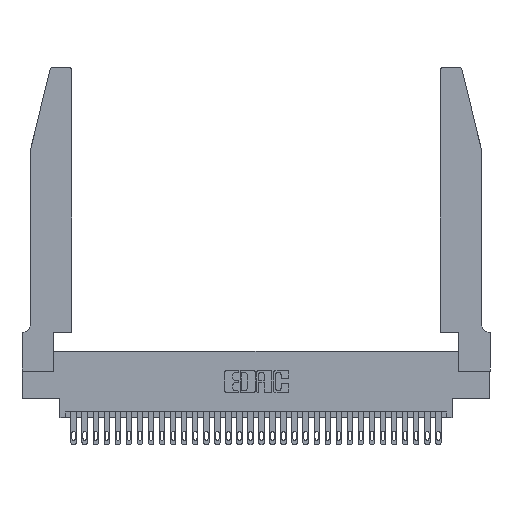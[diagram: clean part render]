
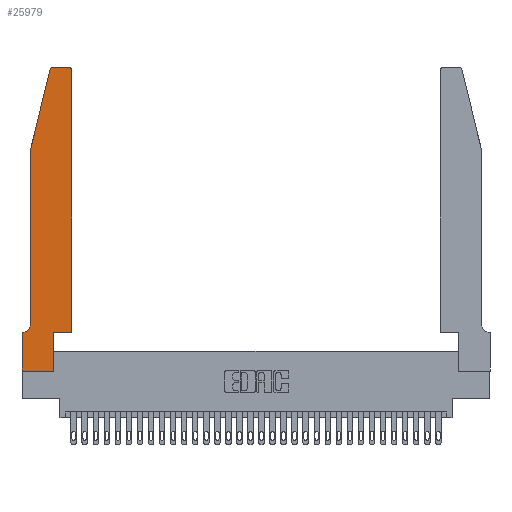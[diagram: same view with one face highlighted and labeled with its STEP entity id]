
A CAD part, top view. The second image highlights one B-rep face of the part: STEP entity #25979.
In plain terms, the highlighted planar face has unit normal (0, 0, 1).
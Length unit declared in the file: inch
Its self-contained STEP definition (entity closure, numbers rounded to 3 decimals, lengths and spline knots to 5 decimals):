
#18 = AXIS2_PLACEMENT_3D ( 'NONE', #23380, #5973, #31330 ) ;
#108 = CARTESIAN_POINT ( 'NONE',  ( 0., 0.35, 0.37 ) ) ;
#519 = VECTOR ( 'NONE', #17162, 39.37008 ) ;
#830 = EDGE_CURVE ( 'NONE', #32472, #28111, #31416, .T. ) ;
#1582 = CARTESIAN_POINT ( 'NONE',  ( 0.0755, 0.42, 0.37 ) ) ;
#1651 = CIRCLE ( 'NONE', #9747, 0.03 ) ;
#1728 = FACE_OUTER_BOUND ( 'NONE', #7332, .T. ) ;
#1952 = DIRECTION ( 'NONE',  ( -0.239, -0.971, 0. ) ) ;
#1981 = ORIENTED_EDGE ( 'NONE', *, *, #26642, .T. ) ;
#2197 = VECTOR ( 'NONE', #7999, 39.37008 ) ;
#3156 = DIRECTION ( 'NONE',  ( 1., 0., 0. ) ) ;
#3219 = VECTOR ( 'NONE', #1952, 39.37008 ) ;
#3643 = LINE ( 'NONE', #12323, #519 ) ;
#3748 = EDGE_CURVE ( 'NONE', #24625, #18290, #3643, .T. ) ;
#3863 = DIRECTION ( 'NONE',  ( 1., 0., 0. ) ) ;
#4399 = ORIENTED_EDGE ( 'NONE', *, *, #4541, .T. ) ;
#4404 = VECTOR ( 'NONE', #6775, 39.37008 ) ;
#4434 = CARTESIAN_POINT ( 'NONE',  ( 0.4205, 2.75, 0.37 ) ) ;
#4541 = EDGE_CURVE ( 'NONE', #13015, #24625, #31202, .T. ) ;
#5353 = DIRECTION ( 'NONE',  ( 1., 0., 0. ) ) ;
#5883 = AXIS2_PLACEMENT_3D ( 'NONE', #24911, #10011, #15133 ) ;
#5973 = DIRECTION ( 'NONE',  ( 0., 0., -1. ) ) ;
#6484 = LINE ( 'NONE', #19993, #23811 ) ;
#6775 = DIRECTION ( 'NONE',  ( -1., 0., 0. ) ) ;
#6852 = VERTEX_POINT ( 'NONE', #23525 ) ;
#6979 = LINE ( 'NONE', #23469, #15241 ) ;
#7052 = EDGE_CURVE ( 'NONE', #8730, #27240, #17762, .T. ) ;
#7332 = EDGE_LOOP ( 'NONE', ( #29798, #22419, #26788, #13953, #1981, #18088, #27158, #4399, #23398, #14567, #21724, #25975 ) ) ;
#7846 = CARTESIAN_POINT ( 'NONE',  ( 0., 0.35, 0.37 ) ) ;
#7999 = DIRECTION ( 'NONE',  ( 1., 0., 0. ) ) ;
#8064 = DIRECTION ( 'NONE',  ( 0., 0., 1. ) ) ;
#8126 = DIRECTION ( 'NONE',  ( 0., -1., 0. ) ) ;
#8561 = CARTESIAN_POINT ( 'NONE',  ( 0.0755, 0.35, 0.37 ) ) ;
#8730 = VERTEX_POINT ( 'NONE', #4434 ) ;
#9747 = AXIS2_PLACEMENT_3D ( 'NONE', #25950, #8064, #3156 ) ;
#10011 = DIRECTION ( 'NONE',  ( 0., 0., 1. ) ) ;
#11423 = EDGE_CURVE ( 'NONE', #18290, #19737, #23828, .T. ) ;
#12323 = CARTESIAN_POINT ( 'NONE',  ( 0.2865, 0.35, 0.37 ) ) ;
#12983 = CARTESIAN_POINT ( 'NONE',  ( 0.0755, 2., 0.37 ) ) ;
#13015 = VERTEX_POINT ( 'NONE', #13806 ) ;
#13100 = CARTESIAN_POINT ( 'NONE',  ( 0.0755, 2., 0.37 ) ) ;
#13135 = EDGE_CURVE ( 'NONE', #6852, #32472, #14250, .T. ) ;
#13806 = CARTESIAN_POINT ( 'NONE',  ( 0., 0., 0.37 ) ) ;
#13953 = ORIENTED_EDGE ( 'NONE', *, *, #830, .T. ) ;
#14250 = LINE ( 'NONE', #26693, #3219 ) ;
#14567 = ORIENTED_EDGE ( 'NONE', *, *, #11423, .T. ) ;
#14790 = CARTESIAN_POINT ( 'NONE',  ( 0.4505, 0.35, 0.37 ) ) ;
#15133 = DIRECTION ( 'NONE',  ( 1., 0., 0. ) ) ;
#15241 = VECTOR ( 'NONE', #18502, 39.37008 ) ;
#17162 = DIRECTION ( 'NONE',  ( 0., 1., 0. ) ) ;
#17653 = VECTOR ( 'NONE', #24004, 39.37008 ) ;
#17762 = LINE ( 'NONE', #24406, #4404 ) ;
#18088 = ORIENTED_EDGE ( 'NONE', *, *, #22628, .T. ) ;
#18158 = EDGE_CURVE ( 'NONE', #27240, #6852, #20638, .T. ) ;
#18290 = VERTEX_POINT ( 'NONE', #22739 ) ;
#18502 = DIRECTION ( 'NONE',  ( 0., -1., 0. ) ) ;
#18814 = VERTEX_POINT ( 'NONE', #28233 ) ;
#19190 = VERTEX_POINT ( 'NONE', #27364 ) ;
#19486 = EDGE_CURVE ( 'NONE', #31900, #13015, #6979, .T. ) ;
#19737 = VERTEX_POINT ( 'NONE', #14790 ) ;
#19993 = CARTESIAN_POINT ( 'NONE',  ( 0.4505, 0.35, 0.37 ) ) ;
#20240 = PLANE ( 'NONE',  #21702 ) ;
#20543 = EDGE_CURVE ( 'NONE', #19190, #8730, #1651, .T. ) ;
#20638 = CIRCLE ( 'NONE', #5883, 0.03 ) ;
#21377 = CARTESIAN_POINT ( 'NONE',  ( 0., 0., 0.37 ) ) ;
#21702 = AXIS2_PLACEMENT_3D ( 'NONE', #108, #30695, #5353 ) ;
#21724 = ORIENTED_EDGE ( 'NONE', *, *, #31769, .T. ) ;
#22236 = CARTESIAN_POINT ( 'NONE',  ( 0.2865, 0., 0.37 ) ) ;
#22419 = ORIENTED_EDGE ( 'NONE', *, *, #18158, .T. ) ;
#22628 = EDGE_CURVE ( 'NONE', #18814, #31900, #25529, .T. ) ;
#22739 = CARTESIAN_POINT ( 'NONE',  ( 0.2865, 0.35, 0.37 ) ) ;
#22896 = CARTESIAN_POINT ( 'NONE',  ( 0.4505, 0.35, 0.37 ) ) ;
#23349 = CIRCLE ( 'NONE', #18, 0.07 ) ;
#23380 = CARTESIAN_POINT ( 'NONE',  ( 0.0055, 0.42, 0.37 ) ) ;
#23398 = ORIENTED_EDGE ( 'NONE', *, *, #3748, .T. ) ;
#23469 = CARTESIAN_POINT ( 'NONE',  ( 0., 0., 0.37 ) ) ;
#23525 = CARTESIAN_POINT ( 'NONE',  ( 0.25487, 2.72718, 0.37 ) ) ;
#23811 = VECTOR ( 'NONE', #27601, 39.37008 ) ;
#23828 = LINE ( 'NONE', #22896, #2197 ) ;
#24004 = DIRECTION ( 'NONE',  ( -1., 0., 0. ) ) ;
#24406 = CARTESIAN_POINT ( 'NONE',  ( 0.2605, 2.75, 0.37 ) ) ;
#24493 = VECTOR ( 'NONE', #3863, 39.37008 ) ;
#24625 = VERTEX_POINT ( 'NONE', #22236 ) ;
#24911 = CARTESIAN_POINT ( 'NONE',  ( 0.284, 2.72, 0.37 ) ) ;
#25529 = LINE ( 'NONE', #8561, #17653 ) ;
#25950 = CARTESIAN_POINT ( 'NONE',  ( 0.4205, 2.72, 0.37 ) ) ;
#25975 = ORIENTED_EDGE ( 'NONE', *, *, #20543, .T. ) ;
#25979 = ADVANCED_FACE ( 'NONE', ( #1728 ), #20240, .T. ) ;
#26642 = EDGE_CURVE ( 'NONE', #28111, #18814, #23349, .T. ) ;
#26693 = CARTESIAN_POINT ( 'NONE',  ( 0.0755, 2., 0.37 ) ) ;
#26788 = ORIENTED_EDGE ( 'NONE', *, *, #13135, .T. ) ;
#27158 = ORIENTED_EDGE ( 'NONE', *, *, #19486, .T. ) ;
#27240 = VERTEX_POINT ( 'NONE', #30627 ) ;
#27364 = CARTESIAN_POINT ( 'NONE',  ( 0.4505, 2.72, 0.37 ) ) ;
#27601 = DIRECTION ( 'NONE',  ( 0., 1., 0. ) ) ;
#28111 = VERTEX_POINT ( 'NONE', #1582 ) ;
#28233 = CARTESIAN_POINT ( 'NONE',  ( 0.0055, 0.35, 0.37 ) ) ;
#29798 = ORIENTED_EDGE ( 'NONE', *, *, #7052, .T. ) ;
#30627 = CARTESIAN_POINT ( 'NONE',  ( 0.284, 2.75, 0.37 ) ) ;
#30695 = DIRECTION ( 'NONE',  ( 0., 0., 1. ) ) ;
#31003 = VECTOR ( 'NONE', #8126, 39.37008 ) ;
#31202 = LINE ( 'NONE', #21377, #24493 ) ;
#31330 = DIRECTION ( 'NONE',  ( -1., 0., 0. ) ) ;
#31416 = LINE ( 'NONE', #13100, #31003 ) ;
#31769 = EDGE_CURVE ( 'NONE', #19737, #19190, #6484, .T. ) ;
#31900 = VERTEX_POINT ( 'NONE', #7846 ) ;
#32472 = VERTEX_POINT ( 'NONE', #12983 ) ;
